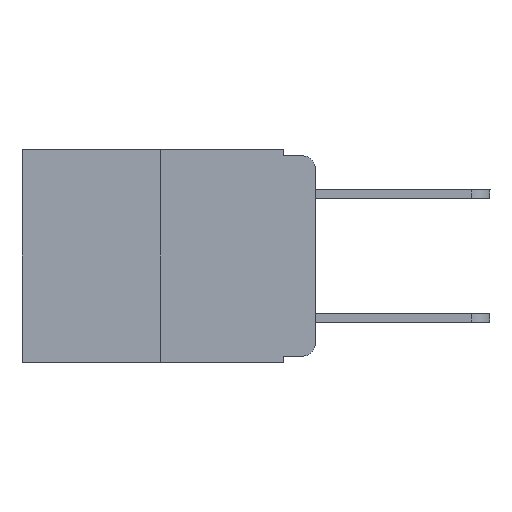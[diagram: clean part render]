
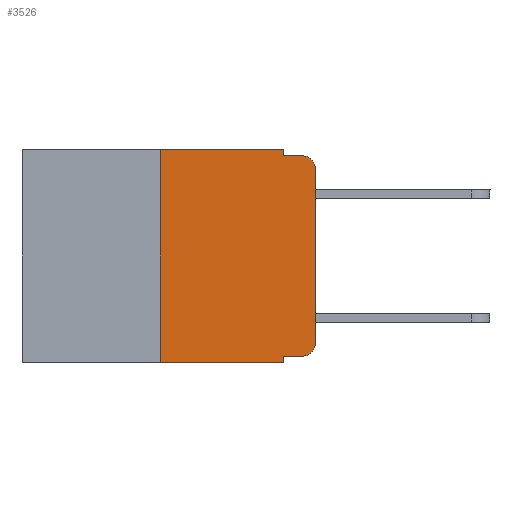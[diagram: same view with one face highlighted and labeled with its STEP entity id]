
A CAD part, left-side view. The second image highlights one B-rep face of the part: STEP entity #3526.
In plain terms, the highlighted planar face has unit normal (-1, 0, 0).
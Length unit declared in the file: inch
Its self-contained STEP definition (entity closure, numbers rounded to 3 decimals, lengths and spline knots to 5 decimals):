
#97 = VECTOR ( 'NONE', #6526, 39.37008 ) ;
#154 = DIRECTION ( 'NONE',  ( 0., 0., -1. ) ) ;
#274 = ORIENTED_EDGE ( 'NONE', *, *, #3060, .T. ) ;
#568 = DIRECTION ( 'NONE',  ( -1., 0., 0. ) ) ;
#622 = AXIS2_PLACEMENT_3D ( 'NONE', #10063, #9881, #11053 ) ;
#668 = CARTESIAN_POINT ( 'NONE',  ( 0., 0.051, -0.01 ) ) ;
#891 = EDGE_CURVE ( 'NONE', #10739, #1089, #11756, .T. ) ;
#952 = ORIENTED_EDGE ( 'NONE', *, *, #10485, .F. ) ;
#1089 = VERTEX_POINT ( 'NONE', #6831 ) ;
#1304 = CARTESIAN_POINT ( 'NONE',  ( 0., 0.02, -0.333 ) ) ;
#1499 = DIRECTION ( 'NONE',  ( 0., -1., 0. ) ) ;
#1512 = VERTEX_POINT ( 'NONE', #10725 ) ;
#1590 = ORIENTED_EDGE ( 'NONE', *, *, #7017, .T. ) ;
#1978 = EDGE_CURVE ( 'NONE', #2480, #6399, #6803, .T. ) ;
#2028 = VECTOR ( 'NONE', #11401, 39.37008 ) ;
#2057 = ORIENTED_EDGE ( 'NONE', *, *, #12478, .T. ) ;
#2186 = EDGE_LOOP ( 'NONE', ( #1590, #2057, #952, #10622, #9237, #2556, #8740, #8510, #274, #10360 ) ) ;
#2399 = VERTEX_POINT ( 'NONE', #7733 ) ;
#2477 = EDGE_CURVE ( 'NONE', #6399, #4754, #3252, .T. ) ;
#2480 = VERTEX_POINT ( 'NONE', #6979 ) ;
#2499 = AXIS2_PLACEMENT_3D ( 'NONE', #11832, #568, #11112 ) ;
#2556 = ORIENTED_EDGE ( 'NONE', *, *, #9620, .F. ) ;
#2557 = LINE ( 'NONE', #7349, #11240 ) ;
#2565 = DIRECTION ( 'NONE',  ( 1., 0., 0. ) ) ;
#3060 = EDGE_CURVE ( 'NONE', #2399, #10739, #12043, .T. ) ;
#3135 = CARTESIAN_POINT ( 'NONE',  ( 0., 0.051, 0. ) ) ;
#3252 = LINE ( 'NONE', #3135, #6764 ) ;
#3519 = DIRECTION ( 'NONE',  ( 0., 0., -1. ) ) ;
#3526 = ADVANCED_FACE ( 'NONE', ( #9382 ), #5474, .F. ) ;
#3567 = DIRECTION ( 'NONE',  ( 0., 0., 1. ) ) ;
#3931 = VERTEX_POINT ( 'NONE', #4642 ) ;
#3971 = EDGE_CURVE ( 'NONE', #6547, #1512, #10427, .T. ) ;
#4400 = VECTOR ( 'NONE', #154, 39.37008 ) ;
#4642 = CARTESIAN_POINT ( 'NONE',  ( 0., 0.02, -0.01 ) ) ;
#4754 = VERTEX_POINT ( 'NONE', #12112 ) ;
#5361 = CARTESIAN_POINT ( 'NONE',  ( 0., 0.051, 0. ) ) ;
#5474 = PLANE ( 'NONE',  #11598 ) ;
#6399 = VERTEX_POINT ( 'NONE', #5361 ) ;
#6526 = DIRECTION ( 'NONE',  ( 0., -1., 0. ) ) ;
#6547 = VERTEX_POINT ( 'NONE', #10322 ) ;
#6554 = VECTOR ( 'NONE', #7817, 39.37008 ) ;
#6641 = CARTESIAN_POINT ( 'NONE',  ( 0., 0.25, 0. ) ) ;
#6682 = EDGE_CURVE ( 'NONE', #2399, #1512, #9882, .T. ) ;
#6764 = VECTOR ( 'NONE', #8169, 39.37008 ) ;
#6803 = LINE ( 'NONE', #10641, #6554 ) ;
#6831 = CARTESIAN_POINT ( 'NONE',  ( 0., 0., -0.313 ) ) ;
#6979 = CARTESIAN_POINT ( 'NONE',  ( 0., 0.25, 0. ) ) ;
#7017 = EDGE_CURVE ( 'NONE', #1089, #12028, #2557, .T. ) ;
#7251 = CARTESIAN_POINT ( 'NONE',  ( 0., 0.051, -0.333 ) ) ;
#7349 = CARTESIAN_POINT ( 'NONE',  ( 0., 0., 0. ) ) ;
#7529 = DIRECTION ( 'NONE',  ( 0., 0., 1. ) ) ;
#7733 = CARTESIAN_POINT ( 'NONE',  ( 0., 0.051, -0.333 ) ) ;
#7817 = DIRECTION ( 'NONE',  ( 0., -1., 0. ) ) ;
#8152 = VECTOR ( 'NONE', #1499, 39.37008 ) ;
#8169 = DIRECTION ( 'NONE',  ( 0., 0., -1. ) ) ;
#8510 = ORIENTED_EDGE ( 'NONE', *, *, #6682, .F. ) ;
#8546 = CARTESIAN_POINT ( 'NONE',  ( 0., 0.473, -0.343 ) ) ;
#8740 = ORIENTED_EDGE ( 'NONE', *, *, #3971, .T. ) ;
#8871 = CARTESIAN_POINT ( 'NONE',  ( 0., 0.051, 0. ) ) ;
#9074 = CARTESIAN_POINT ( 'NONE',  ( 0., 0., -0.03 ) ) ;
#9237 = ORIENTED_EDGE ( 'NONE', *, *, #1978, .F. ) ;
#9382 = FACE_OUTER_BOUND ( 'NONE', #2186, .T. ) ;
#9620 = EDGE_CURVE ( 'NONE', #6547, #2480, #11305, .T. ) ;
#9881 = DIRECTION ( 'NONE',  ( -1., 0., 0. ) ) ;
#9882 = LINE ( 'NONE', #8871, #4400 ) ;
#10063 = CARTESIAN_POINT ( 'NONE',  ( 0., 0.02, -0.03 ) ) ;
#10318 = CARTESIAN_POINT ( 'NONE',  ( 0., 0.473, 0. ) ) ;
#10322 = CARTESIAN_POINT ( 'NONE',  ( 0., 0.25, -0.343 ) ) ;
#10360 = ORIENTED_EDGE ( 'NONE', *, *, #891, .T. ) ;
#10427 = LINE ( 'NONE', #8546, #97 ) ;
#10485 = EDGE_CURVE ( 'NONE', #4754, #3931, #12287, .T. ) ;
#10622 = ORIENTED_EDGE ( 'NONE', *, *, #2477, .F. ) ;
#10641 = CARTESIAN_POINT ( 'NONE',  ( 0., 0.473, 0. ) ) ;
#10725 = CARTESIAN_POINT ( 'NONE',  ( 0., 0.051, -0.343 ) ) ;
#10739 = VERTEX_POINT ( 'NONE', #1304 ) ;
#11053 = DIRECTION ( 'NONE',  ( 0., 0., -1. ) ) ;
#11112 = DIRECTION ( 'NONE',  ( 0., 0., -1. ) ) ;
#11240 = VECTOR ( 'NONE', #3567, 39.37008 ) ;
#11305 = LINE ( 'NONE', #6641, #12073 ) ;
#11401 = DIRECTION ( 'NONE',  ( 0., -1., 0. ) ) ;
#11598 = AXIS2_PLACEMENT_3D ( 'NONE', #10318, #2565, #3519 ) ;
#11756 = CIRCLE ( 'NONE', #2499, 0.02 ) ;
#11832 = CARTESIAN_POINT ( 'NONE',  ( 0., 0.02, -0.313 ) ) ;
#11926 = CIRCLE ( 'NONE', #622, 0.02 ) ;
#12028 = VERTEX_POINT ( 'NONE', #9074 ) ;
#12043 = LINE ( 'NONE', #7251, #8152 ) ;
#12073 = VECTOR ( 'NONE', #7529, 39.37008 ) ;
#12112 = CARTESIAN_POINT ( 'NONE',  ( 0., 0.051, -0.01 ) ) ;
#12287 = LINE ( 'NONE', #668, #2028 ) ;
#12478 = EDGE_CURVE ( 'NONE', #12028, #3931, #11926, .T. ) ;
